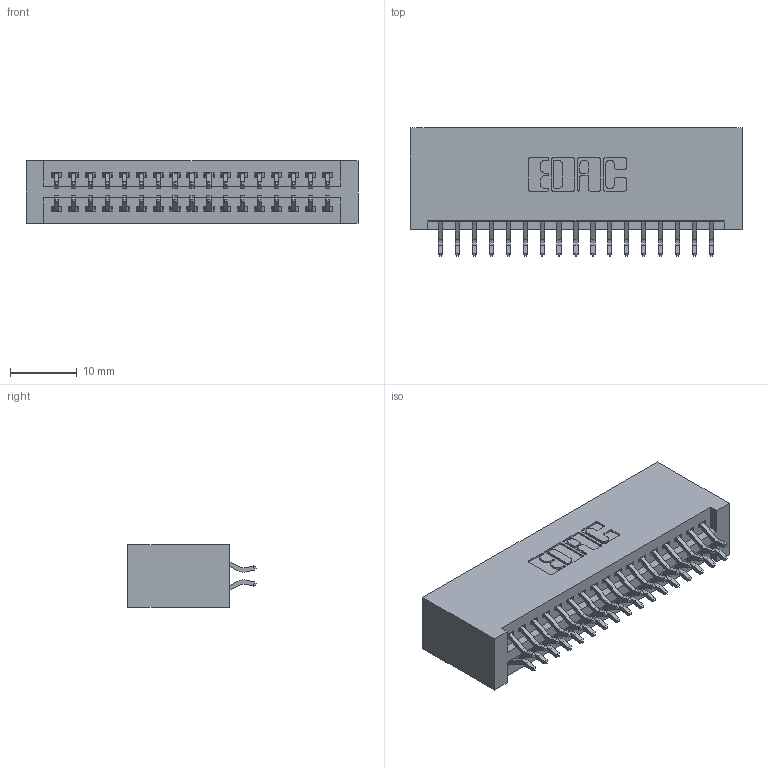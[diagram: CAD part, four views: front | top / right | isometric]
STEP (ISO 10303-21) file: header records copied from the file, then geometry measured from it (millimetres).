
FILE_DESCRIPTION (( 'STEP AP203' ), '1' );
FILE_NAME ('345-034-556-201.STEP', '2018-08-29T03:49:05', ( '' ), ( '' ), 'SwSTEP 2.0', 'SolidWorks 2016', '' );
FILE_SCHEMA (( 'CONFIG_CONTROL_DESIGN' ));
Length unit declared in the file: inch
Products named in the file (3): 345-292-001_556 Tail; 345-034-556-201; 345 Part_No Mounting Lugs
Assembly tree (35 placements, depth 2):
  345-034-556-201
    345 Part_No Mounting Lugs
    345-292-001_556 Tail  x34
Bounding box: 49.78 x 19.24 x 9.4 mm (x, y, z)
Volume: 5218.6 mm3; surface area: 7503.2 mm2
Topology: 35 solids, 35 shells, 2022 faces, 5995 edges, 3950 vertices
Faces by surface type: plane 1334, cylinder 688
Entity records: 16647 total; most frequent: CARTESIAN_POINT 2828, ORIENTED_EDGE 2750, DIRECTION 2507, EDGE_CURVE 1375, LINE 1175, VECTOR 1175, VERTEX_POINT 914, AXIS2_PLACEMENT_3D 666
